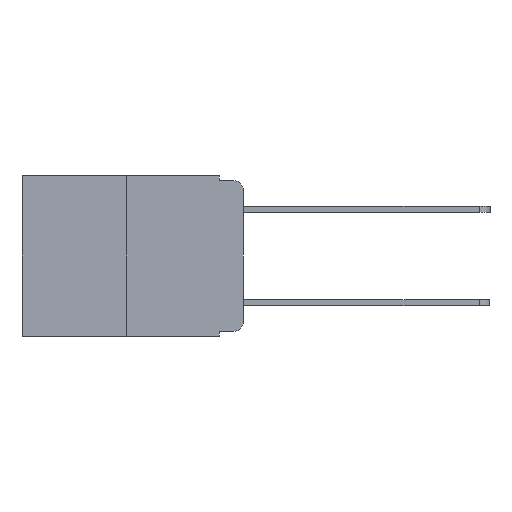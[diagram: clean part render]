
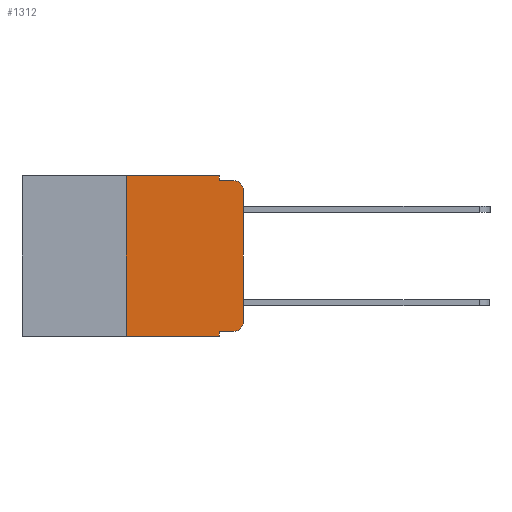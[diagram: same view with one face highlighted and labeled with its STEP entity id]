
A CAD part, left-side view. The second image highlights one B-rep face of the part: STEP entity #1312.
In plain terms, the highlighted planar face has unit normal (-1, 0, 0).
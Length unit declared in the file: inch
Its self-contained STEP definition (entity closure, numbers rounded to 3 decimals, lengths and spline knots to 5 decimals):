
#59 = CARTESIAN_POINT ( 'NONE',  ( 0., 0.051, 0. ) ) ;
#93 = CARTESIAN_POINT ( 'NONE',  ( 0., 0.051, -0.01 ) ) ;
#238 = ORIENTED_EDGE ( 'NONE', *, *, #6407, .F. ) ;
#247 = ORIENTED_EDGE ( 'NONE', *, *, #5885, .T. ) ;
#266 = ORIENTED_EDGE ( 'NONE', *, *, #7845, .F. ) ;
#364 = CARTESIAN_POINT ( 'NONE',  ( 0., 0.051, -0.333 ) ) ;
#511 = ORIENTED_EDGE ( 'NONE', *, *, #5086, .F. ) ;
#771 = EDGE_CURVE ( 'NONE', #9858, #4947, #9116, .T. ) ;
#914 = LINE ( 'NONE', #8317, #8972 ) ;
#1312 = ADVANCED_FACE ( 'NONE', ( #4090 ), #3791, .F. ) ;
#1323 = CARTESIAN_POINT ( 'NONE',  ( 0., 0.02, -0.03 ) ) ;
#1608 = DIRECTION ( 'NONE',  ( -1., 0., 0. ) ) ;
#1811 = ORIENTED_EDGE ( 'NONE', *, *, #4298, .T. ) ;
#1852 = ORIENTED_EDGE ( 'NONE', *, *, #8314, .F. ) ;
#1901 = CIRCLE ( 'NONE', #9494, 0.02 ) ;
#1921 = ORIENTED_EDGE ( 'NONE', *, *, #771, .T. ) ;
#1930 = ORIENTED_EDGE ( 'NONE', *, *, #9276, .F. ) ;
#2018 = ORIENTED_EDGE ( 'NONE', *, *, #2497, .T. ) ;
#2232 = DIRECTION ( 'NONE',  ( 0., 0., -1. ) ) ;
#2278 = DIRECTION ( 'NONE',  ( 0., -1., 0. ) ) ;
#2321 = LINE ( 'NONE', #59, #8183 ) ;
#2497 = EDGE_CURVE ( 'NONE', #5002, #5868, #9473, .T. ) ;
#2517 = ORIENTED_EDGE ( 'NONE', *, *, #3582, .T. ) ;
#2566 = VECTOR ( 'NONE', #7251, 39.37008 ) ;
#2832 = DIRECTION ( 'NONE',  ( 0., 0., -1. ) ) ;
#3476 = CARTESIAN_POINT ( 'NONE',  ( 0., 0.02, -0.313 ) ) ;
#3582 = EDGE_CURVE ( 'NONE', #5868, #6047, #4705, .T. ) ;
#3791 = PLANE ( 'NONE',  #8353 ) ;
#4090 = FACE_OUTER_BOUND ( 'NONE', #9462, .T. ) ;
#4294 = VERTEX_POINT ( 'NONE', #4898 ) ;
#4298 = EDGE_CURVE ( 'NONE', #6047, #7620, #8313, .T. ) ;
#4302 = DIRECTION ( 'NONE',  ( 1., 0., 0. ) ) ;
#4361 = VERTEX_POINT ( 'NONE', #8214 ) ;
#4368 = VERTEX_POINT ( 'NONE', #9349 ) ;
#4379 = CARTESIAN_POINT ( 'NONE',  ( 0., 0.25, -0.343 ) ) ;
#4705 = CIRCLE ( 'NONE', #9147, 0.02 ) ;
#4898 = CARTESIAN_POINT ( 'NONE',  ( 0., 0.02, -0.01 ) ) ;
#4907 = LINE ( 'NONE', #4943, #2566 ) ;
#4943 = CARTESIAN_POINT ( 'NONE',  ( 0., 0.25, 0. ) ) ;
#4947 = VERTEX_POINT ( 'NONE', #6410 ) ;
#5002 = VERTEX_POINT ( 'NONE', #9854 ) ;
#5086 = EDGE_CURVE ( 'NONE', #4368, #8799, #914, .T. ) ;
#5348 = VECTOR ( 'NONE', #7950, 39.37008 ) ;
#5576 = CARTESIAN_POINT ( 'NONE',  ( 0., 0.473, 0. ) ) ;
#5688 = CARTESIAN_POINT ( 'NONE',  ( 0., 0., -0.03 ) ) ;
#5868 = VERTEX_POINT ( 'NONE', #9731 ) ;
#5885 = EDGE_CURVE ( 'NONE', #7620, #4294, #1901, .T. ) ;
#5886 = CARTESIAN_POINT ( 'NONE',  ( 0., 0.473, -0.343 ) ) ;
#5912 = DIRECTION ( 'NONE',  ( 0., 0., -1. ) ) ;
#5997 = DIRECTION ( 'NONE',  ( 0., -1., 0. ) ) ;
#6015 = VECTOR ( 'NONE', #5912, 39.37008 ) ;
#6047 = VERTEX_POINT ( 'NONE', #9213 ) ;
#6407 = EDGE_CURVE ( 'NONE', #4361, #4294, #8594, .T. ) ;
#6410 = CARTESIAN_POINT ( 'NONE',  ( 0., 0.051, -0.343 ) ) ;
#6418 = VECTOR ( 'NONE', #7104, 39.37008 ) ;
#6714 = VECTOR ( 'NONE', #5997, 39.37008 ) ;
#6917 = DIRECTION ( 'NONE',  ( -1., 0., 0. ) ) ;
#7104 = DIRECTION ( 'NONE',  ( 0., 0., 1. ) ) ;
#7209 = VECTOR ( 'NONE', #8452, 39.37008 ) ;
#7251 = DIRECTION ( 'NONE',  ( 0., 0., 1. ) ) ;
#7620 = VERTEX_POINT ( 'NONE', #5688 ) ;
#7845 = EDGE_CURVE ( 'NONE', #8799, #4361, #2321, .T. ) ;
#7945 = LINE ( 'NONE', #8786, #6015 ) ;
#7950 = DIRECTION ( 'NONE',  ( 0., -1., 0. ) ) ;
#8150 = DIRECTION ( 'NONE',  ( 0., 0., -1. ) ) ;
#8183 = VECTOR ( 'NONE', #8150, 39.37008 ) ;
#8214 = CARTESIAN_POINT ( 'NONE',  ( 0., 0.051, -0.01 ) ) ;
#8297 = CARTESIAN_POINT ( 'NONE',  ( 0., 0.051, 0. ) ) ;
#8313 = LINE ( 'NONE', #8686, #6418 ) ;
#8314 = EDGE_CURVE ( 'NONE', #9858, #4368, #4907, .T. ) ;
#8317 = CARTESIAN_POINT ( 'NONE',  ( 0., 0.473, 0. ) ) ;
#8348 = DIRECTION ( 'NONE',  ( 0., 0., -1. ) ) ;
#8353 = AXIS2_PLACEMENT_3D ( 'NONE', #5576, #4302, #8348 ) ;
#8452 = DIRECTION ( 'NONE',  ( 0., -1., 0. ) ) ;
#8594 = LINE ( 'NONE', #93, #6714 ) ;
#8686 = CARTESIAN_POINT ( 'NONE',  ( 0., 0., 0. ) ) ;
#8786 = CARTESIAN_POINT ( 'NONE',  ( 0., 0.051, 0. ) ) ;
#8799 = VERTEX_POINT ( 'NONE', #8297 ) ;
#8972 = VECTOR ( 'NONE', #2278, 39.37008 ) ;
#9116 = LINE ( 'NONE', #5886, #7209 ) ;
#9147 = AXIS2_PLACEMENT_3D ( 'NONE', #3476, #1608, #2832 ) ;
#9213 = CARTESIAN_POINT ( 'NONE',  ( 0., 0., -0.313 ) ) ;
#9276 = EDGE_CURVE ( 'NONE', #5002, #4947, #7945, .T. ) ;
#9349 = CARTESIAN_POINT ( 'NONE',  ( 0., 0.25, 0. ) ) ;
#9462 = EDGE_LOOP ( 'NONE', ( #1811, #247, #238, #266, #511, #1852, #1921, #1930, #2018, #2517 ) ) ;
#9473 = LINE ( 'NONE', #364, #5348 ) ;
#9494 = AXIS2_PLACEMENT_3D ( 'NONE', #1323, #6917, #2232 ) ;
#9731 = CARTESIAN_POINT ( 'NONE',  ( 0., 0.02, -0.333 ) ) ;
#9854 = CARTESIAN_POINT ( 'NONE',  ( 0., 0.051, -0.333 ) ) ;
#9858 = VERTEX_POINT ( 'NONE', #4379 ) ;
